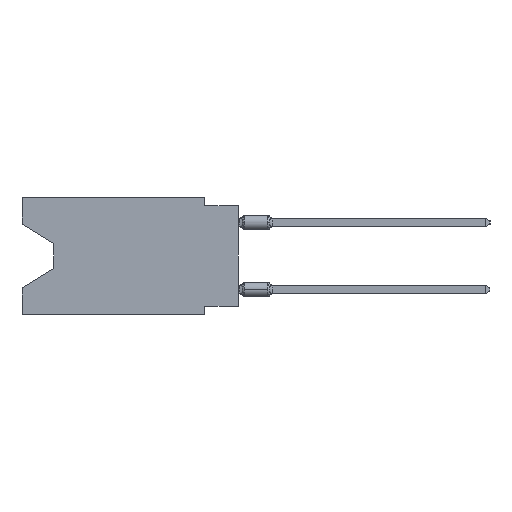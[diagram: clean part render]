
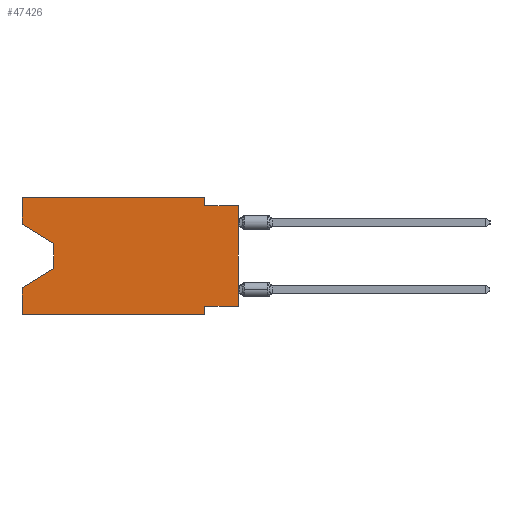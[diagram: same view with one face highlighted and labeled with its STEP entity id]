
A CAD part, left-side view. The second image highlights one B-rep face of the part: STEP entity #47426.
In plain terms, the highlighted planar face has unit normal (-1, 0, 0).
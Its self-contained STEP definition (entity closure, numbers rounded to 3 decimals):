
#848 = LINE ( 'NONE', #5621, #57691 ) ;
#1527 = CARTESIAN_POINT ( 'NONE',  ( 0., 13.97, -3.505 ) ) ;
#2391 = CARTESIAN_POINT ( 'NONE',  ( 0., 2.54, 0. ) ) ;
#3474 = CARTESIAN_POINT ( 'NONE',  ( 0., 16.383, -2.038 ) ) ;
#3730 = LINE ( 'NONE', #42349, #38460 ) ;
#3816 = ORIENTED_EDGE ( 'NONE', *, *, #11174, .F. ) ;
#4200 = EDGE_CURVE ( 'NONE', #43070, #31996, #47558, .T. ) ;
#5104 = DIRECTION ( 'NONE',  ( 1., 0., 0. ) ) ;
#5621 = CARTESIAN_POINT ( 'NONE',  ( 0., 16.383, 0. ) ) ;
#6286 = EDGE_CURVE ( 'NONE', #51286, #38462, #27012, .T. ) ;
#7186 = CARTESIAN_POINT ( 'NONE',  ( 0., 2.54, -8.255 ) ) ;
#7369 = LINE ( 'NONE', #3474, #25610 ) ;
#7586 = EDGE_CURVE ( 'NONE', #43070, #22816, #18672, .T. ) ;
#7755 = ORIENTED_EDGE ( 'NONE', *, *, #57312, .F. ) ;
#8583 = DIRECTION ( 'NONE',  ( 0., 0., -1. ) ) ;
#9175 = CARTESIAN_POINT ( 'NONE',  ( 0., 16.383, 0. ) ) ;
#9205 = AXIS2_PLACEMENT_3D ( 'NONE', #61798, #5104, #19365 ) ;
#9447 = CARTESIAN_POINT ( 'NONE',  ( 0., 13.97, -5.385 ) ) ;
#11010 = ORIENTED_EDGE ( 'NONE', *, *, #53915, .F. ) ;
#11174 = EDGE_CURVE ( 'NONE', #13574, #43008, #19194, .T. ) ;
#11314 = DIRECTION ( 'NONE',  ( 0., -1., 0. ) ) ;
#12943 = ORIENTED_EDGE ( 'NONE', *, *, #17275, .T. ) ;
#13574 = VERTEX_POINT ( 'NONE', #2391 ) ;
#14137 = DIRECTION ( 'NONE',  ( 0., 0., -1. ) ) ;
#15883 = ORIENTED_EDGE ( 'NONE', *, *, #6286, .T. ) ;
#16506 = ORIENTED_EDGE ( 'NONE', *, *, #52819, .F. ) ;
#16970 = DIRECTION ( 'NONE',  ( 0., -1., 0. ) ) ;
#17275 = EDGE_CURVE ( 'NONE', #19753, #21067, #7369, .T. ) ;
#18184 = EDGE_CURVE ( 'NONE', #19753, #52869, #24650, .T. ) ;
#18437 = DIRECTION ( 'NONE',  ( 0., -1., 0. ) ) ;
#18672 = LINE ( 'NONE', #9175, #44178 ) ;
#19194 = LINE ( 'NONE', #62573, #34215 ) ;
#19365 = DIRECTION ( 'NONE',  ( 0., 0., -1. ) ) ;
#19644 = VECTOR ( 'NONE', #39191, 1000. ) ;
#19753 = VERTEX_POINT ( 'NONE', #47526 ) ;
#21067 = VERTEX_POINT ( 'NONE', #1527 ) ;
#21299 = DIRECTION ( 'NONE',  ( 0., -0.855, -0.519 ) ) ;
#22575 = CARTESIAN_POINT ( 'NONE',  ( 0., 2.54, -0.635 ) ) ;
#22740 = ORIENTED_EDGE ( 'NONE', *, *, #29260, .F. ) ;
#22816 = VERTEX_POINT ( 'NONE', #42381 ) ;
#24073 = DIRECTION ( 'NONE',  ( 0., 0., -1. ) ) ;
#24650 = LINE ( 'NONE', #33524, #19644 ) ;
#24859 = VECTOR ( 'NONE', #8583, 1000. ) ;
#25066 = CARTESIAN_POINT ( 'NONE',  ( 0., 16.383, -8.89 ) ) ;
#25610 = VECTOR ( 'NONE', #21299, 1000. ) ;
#27012 = LINE ( 'NONE', #31770, #60263 ) ;
#27252 = ORIENTED_EDGE ( 'NONE', *, *, #62156, .T. ) ;
#28038 = ORIENTED_EDGE ( 'NONE', *, *, #61564, .T. ) ;
#28498 = DIRECTION ( 'NONE',  ( 0., 0., 1. ) ) ;
#29004 = CARTESIAN_POINT ( 'NONE',  ( 0., 0., -0.635 ) ) ;
#29130 = LINE ( 'NONE', #38012, #58501 ) ;
#29155 = FACE_OUTER_BOUND ( 'NONE', #42428, .T. ) ;
#29204 = CARTESIAN_POINT ( 'NONE',  ( 0., 2.54, -8.89 ) ) ;
#29260 = EDGE_CURVE ( 'NONE', #52869, #13574, #848, .T. ) ;
#31770 = CARTESIAN_POINT ( 'NONE',  ( 0., 0., 0. ) ) ;
#31996 = VERTEX_POINT ( 'NONE', #29204 ) ;
#33524 = CARTESIAN_POINT ( 'NONE',  ( 0., 16.383, 0. ) ) ;
#34215 = VECTOR ( 'NONE', #14137, 1000. ) ;
#34611 = VECTOR ( 'NONE', #18437, 1000. ) ;
#36379 = VECTOR ( 'NONE', #16970, 1000. ) ;
#37731 = PLANE ( 'NONE',  #9205 ) ;
#38012 = CARTESIAN_POINT ( 'NONE',  ( 0., 2.54, -8.89 ) ) ;
#38460 = VECTOR ( 'NONE', #61667, 1000. ) ;
#38462 = VERTEX_POINT ( 'NONE', #29004 ) ;
#38933 = ORIENTED_EDGE ( 'NONE', *, *, #4200, .T. ) ;
#39044 = CARTESIAN_POINT ( 'NONE',  ( 0., 13.97, -5.385 ) ) ;
#39191 = DIRECTION ( 'NONE',  ( 0., 0., 1. ) ) ;
#42132 = ORIENTED_EDGE ( 'NONE', *, *, #18184, .F. ) ;
#42349 = CARTESIAN_POINT ( 'NONE',  ( 0., 0., -8.255 ) ) ;
#42381 = CARTESIAN_POINT ( 'NONE',  ( 0., 16.383, -6.852 ) ) ;
#42428 = EDGE_LOOP ( 'NONE', ( #12943, #28038, #27252, #52272, #38933, #7755, #16506, #15883, #11010, #3816, #22740, #42132 ) ) ;
#42820 = CARTESIAN_POINT ( 'NONE',  ( 0., 16.383, -8.89 ) ) ;
#43008 = VERTEX_POINT ( 'NONE', #22575 ) ;
#43070 = VERTEX_POINT ( 'NONE', #25066 ) ;
#43308 = DIRECTION ( 'NONE',  ( 0., 0.855, -0.519 ) ) ;
#43944 = CARTESIAN_POINT ( 'NONE',  ( 0., 16.383, 0. ) ) ;
#44178 = VECTOR ( 'NONE', #28498, 1000. ) ;
#45824 = VERTEX_POINT ( 'NONE', #39044 ) ;
#46149 = VECTOR ( 'NONE', #43308, 1000. ) ;
#46331 = DIRECTION ( 'NONE',  ( 0., 0., 1. ) ) ;
#47426 = ADVANCED_FACE ( 'NONE', ( #29155 ), #37731, .F. ) ;
#47526 = CARTESIAN_POINT ( 'NONE',  ( 0., 16.383, -2.038 ) ) ;
#47558 = LINE ( 'NONE', #42820, #34611 ) ;
#48776 = CARTESIAN_POINT ( 'NONE',  ( 0., 0., -8.255 ) ) ;
#50742 = LINE ( 'NONE', #51345, #24859 ) ;
#51286 = VERTEX_POINT ( 'NONE', #48776 ) ;
#51345 = CARTESIAN_POINT ( 'NONE',  ( 0., 13.97, -3.505 ) ) ;
#52272 = ORIENTED_EDGE ( 'NONE', *, *, #7586, .F. ) ;
#52819 = EDGE_CURVE ( 'NONE', #51286, #58036, #3730, .T. ) ;
#52869 = VERTEX_POINT ( 'NONE', #43944 ) ;
#53915 = EDGE_CURVE ( 'NONE', #43008, #38462, #60348, .T. ) ;
#56532 = CARTESIAN_POINT ( 'NONE',  ( 0., 0., -0.635 ) ) ;
#56958 = LINE ( 'NONE', #9447, #46149 ) ;
#57312 = EDGE_CURVE ( 'NONE', #58036, #31996, #29130, .T. ) ;
#57691 = VECTOR ( 'NONE', #11314, 1000. ) ;
#58036 = VERTEX_POINT ( 'NONE', #7186 ) ;
#58501 = VECTOR ( 'NONE', #24073, 1000. ) ;
#60263 = VECTOR ( 'NONE', #46331, 1000. ) ;
#60348 = LINE ( 'NONE', #56532, #36379 ) ;
#61564 = EDGE_CURVE ( 'NONE', #21067, #45824, #50742, .T. ) ;
#61667 = DIRECTION ( 'NONE',  ( 0., 1., 0. ) ) ;
#61798 = CARTESIAN_POINT ( 'NONE',  ( 0., 16.383, 0. ) ) ;
#62156 = EDGE_CURVE ( 'NONE', #45824, #22816, #56958, .T. ) ;
#62573 = CARTESIAN_POINT ( 'NONE',  ( 0., 2.54, 0. ) ) ;
